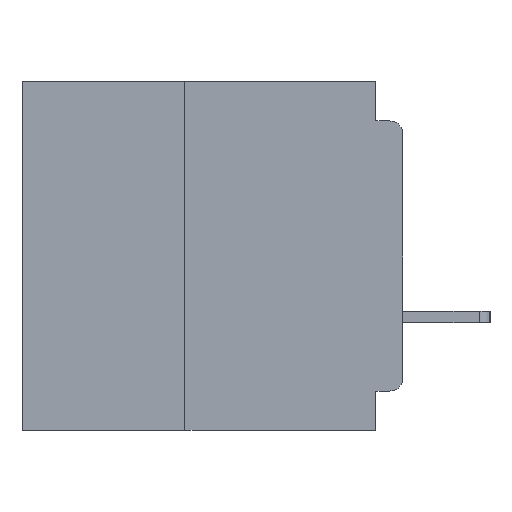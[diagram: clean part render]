
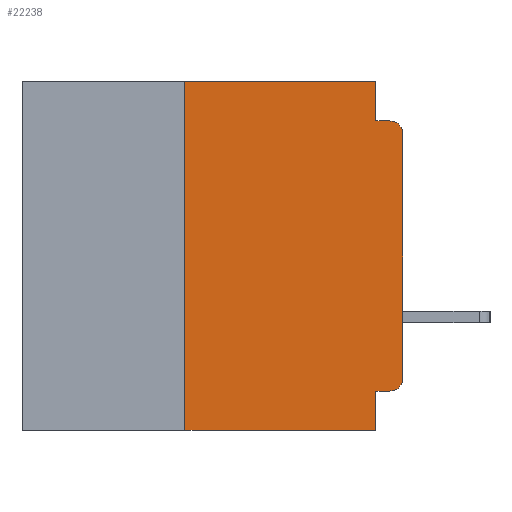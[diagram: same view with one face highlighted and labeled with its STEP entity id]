
A CAD part, left-side view. The second image highlights one B-rep face of the part: STEP entity #22238.
In plain terms, the highlighted planar face has unit normal (-1, 0, 0).
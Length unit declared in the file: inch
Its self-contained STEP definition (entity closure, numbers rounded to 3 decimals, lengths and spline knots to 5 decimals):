
#2017 = CARTESIAN_POINT ( 'NONE',  ( 0., 0., -0.045 ) ) ;
#2453 = DIRECTION ( 'NONE',  ( 0., 0., -1. ) ) ;
#2510 = VECTOR ( 'NONE', #8311, 39.37008 ) ;
#2753 = LINE ( 'NONE', #11465, #4921 ) ;
#3020 = VERTEX_POINT ( 'NONE', #9635 ) ;
#3925 = PLANE ( 'NONE',  #15052 ) ;
#4724 = CIRCLE ( 'NONE', #27396, 0.015 ) ;
#4921 = VECTOR ( 'NONE', #18078, 39.37008 ) ;
#5508 = DIRECTION ( 'NONE',  ( 0., -1., 0. ) ) ;
#5582 = DIRECTION ( 'NONE',  ( -1., 0., 0. ) ) ;
#5783 = VERTEX_POINT ( 'NONE', #24208 ) ;
#5789 = DIRECTION ( 'NONE',  ( 0., 0., 1. ) ) ;
#5846 = VERTEX_POINT ( 'NONE', #14670 ) ;
#5881 = ORIENTED_EDGE ( 'NONE', *, *, #14215, .F. ) ;
#5890 = EDGE_LOOP ( 'NONE', ( #24073, #16083, #37599, #33287, #23704, #41129, #30030, #11794, #5881, #34738 ) ) ;
#6093 = CARTESIAN_POINT ( 'NONE',  ( 0., 0.031, -0.4 ) ) ;
#6143 = VERTEX_POINT ( 'NONE', #19419 ) ;
#6516 = LINE ( 'NONE', #2017, #31098 ) ;
#6546 = CARTESIAN_POINT ( 'NONE',  ( 0., 0.031, -0.045 ) ) ;
#8311 = DIRECTION ( 'NONE',  ( 0., 0., 1. ) ) ;
#8723 = FACE_OUTER_BOUND ( 'NONE', #5890, .T. ) ;
#9014 = LINE ( 'NONE', #33166, #33476 ) ;
#9048 = VECTOR ( 'NONE', #36229, 39.37008 ) ;
#9635 = CARTESIAN_POINT ( 'NONE',  ( 0., 0.25, 0. ) ) ;
#11465 = CARTESIAN_POINT ( 'NONE',  ( 0., 0.031, 0. ) ) ;
#11794 = ORIENTED_EDGE ( 'NONE', *, *, #38532, .F. ) ;
#12131 = EDGE_CURVE ( 'NONE', #6143, #13682, #2753, .T. ) ;
#12743 = EDGE_CURVE ( 'NONE', #35463, #5783, #14540, .T. ) ;
#12857 = CARTESIAN_POINT ( 'NONE',  ( 0., 0.015, -0.355 ) ) ;
#13131 = CARTESIAN_POINT ( 'NONE',  ( 0., 0., -0.355 ) ) ;
#13379 = DIRECTION ( 'NONE',  ( 0., -1., 0. ) ) ;
#13682 = VERTEX_POINT ( 'NONE', #6546 ) ;
#13847 = LINE ( 'NONE', #6093, #38075 ) ;
#14215 = EDGE_CURVE ( 'NONE', #18330, #42657, #34510, .T. ) ;
#14540 = LINE ( 'NONE', #27995, #23322 ) ;
#14670 = CARTESIAN_POINT ( 'NONE',  ( 0., 0., -0.34 ) ) ;
#15052 = AXIS2_PLACEMENT_3D ( 'NONE', #20822, #40639, #20963 ) ;
#15997 = CARTESIAN_POINT ( 'NONE',  ( 0., 0.25, -0.4 ) ) ;
#16083 = ORIENTED_EDGE ( 'NONE', *, *, #27600, .T. ) ;
#18078 = DIRECTION ( 'NONE',  ( 0., 0., -1. ) ) ;
#18118 = DIRECTION ( 'NONE',  ( -1., 0., 0. ) ) ;
#18330 = VERTEX_POINT ( 'NONE', #12857 ) ;
#19281 = CARTESIAN_POINT ( 'NONE',  ( 0., 0., -0.06 ) ) ;
#19416 = CARTESIAN_POINT ( 'NONE',  ( 0., 0.25, -0.4 ) ) ;
#19419 = CARTESIAN_POINT ( 'NONE',  ( 0., 0.031, 0. ) ) ;
#19850 = CIRCLE ( 'NONE', #30784, 0.015 ) ;
#20822 = CARTESIAN_POINT ( 'NONE',  ( 0., 0.437, 0. ) ) ;
#20963 = DIRECTION ( 'NONE',  ( 0., 0., -1. ) ) ;
#21012 = CARTESIAN_POINT ( 'NONE',  ( 0., 0.015, -0.045 ) ) ;
#21649 = VERTEX_POINT ( 'NONE', #21012 ) ;
#22238 = ADVANCED_FACE ( 'NONE', ( #8723 ), #3925, .F. ) ;
#22666 = VECTOR ( 'NONE', #5789, 39.37008 ) ;
#23322 = VECTOR ( 'NONE', #37881, 39.37008 ) ;
#23675 = LINE ( 'NONE', #19416, #22666 ) ;
#23704 = ORIENTED_EDGE ( 'NONE', *, *, #28981, .F. ) ;
#24073 = ORIENTED_EDGE ( 'NONE', *, *, #24654, .T. ) ;
#24208 = CARTESIAN_POINT ( 'NONE',  ( 0., 0.031, -0.4 ) ) ;
#24654 = EDGE_CURVE ( 'NONE', #5846, #38466, #39092, .T. ) ;
#25007 = CARTESIAN_POINT ( 'NONE',  ( 0., 0., 0. ) ) ;
#25696 = CARTESIAN_POINT ( 'NONE',  ( 0., 0.015, -0.34 ) ) ;
#27396 = AXIS2_PLACEMENT_3D ( 'NONE', #25696, #5582, #29031 ) ;
#27600 = EDGE_CURVE ( 'NONE', #38466, #21649, #19850, .T. ) ;
#27995 = CARTESIAN_POINT ( 'NONE',  ( 0., 0.437, -0.4 ) ) ;
#28981 = EDGE_CURVE ( 'NONE', #3020, #6143, #9014, .T. ) ;
#29031 = DIRECTION ( 'NONE',  ( 0., 0., -1. ) ) ;
#30030 = ORIENTED_EDGE ( 'NONE', *, *, #12743, .T. ) ;
#30784 = AXIS2_PLACEMENT_3D ( 'NONE', #37837, #18118, #41126 ) ;
#31098 = VECTOR ( 'NONE', #5508, 39.37008 ) ;
#33166 = CARTESIAN_POINT ( 'NONE',  ( 0., 0.437, 0. ) ) ;
#33287 = ORIENTED_EDGE ( 'NONE', *, *, #12131, .F. ) ;
#33476 = VECTOR ( 'NONE', #13379, 39.37008 ) ;
#34510 = LINE ( 'NONE', #13131, #9048 ) ;
#34738 = ORIENTED_EDGE ( 'NONE', *, *, #43169, .T. ) ;
#35463 = VERTEX_POINT ( 'NONE', #15997 ) ;
#35953 = CARTESIAN_POINT ( 'NONE',  ( 0., 0.031, -0.355 ) ) ;
#36006 = EDGE_CURVE ( 'NONE', #13682, #21649, #6516, .T. ) ;
#36229 = DIRECTION ( 'NONE',  ( 0., 1., 0. ) ) ;
#37599 = ORIENTED_EDGE ( 'NONE', *, *, #36006, .F. ) ;
#37837 = CARTESIAN_POINT ( 'NONE',  ( 0., 0.015, -0.06 ) ) ;
#37881 = DIRECTION ( 'NONE',  ( 0., -1., 0. ) ) ;
#38075 = VECTOR ( 'NONE', #2453, 39.37008 ) ;
#38466 = VERTEX_POINT ( 'NONE', #19281 ) ;
#38498 = EDGE_CURVE ( 'NONE', #35463, #3020, #23675, .T. ) ;
#38532 = EDGE_CURVE ( 'NONE', #42657, #5783, #13847, .T. ) ;
#39092 = LINE ( 'NONE', #25007, #2510 ) ;
#40639 = DIRECTION ( 'NONE',  ( 1., 0., 0. ) ) ;
#41126 = DIRECTION ( 'NONE',  ( 0., 0., -1. ) ) ;
#41129 = ORIENTED_EDGE ( 'NONE', *, *, #38498, .F. ) ;
#42657 = VERTEX_POINT ( 'NONE', #35953 ) ;
#43169 = EDGE_CURVE ( 'NONE', #18330, #5846, #4724, .T. ) ;
